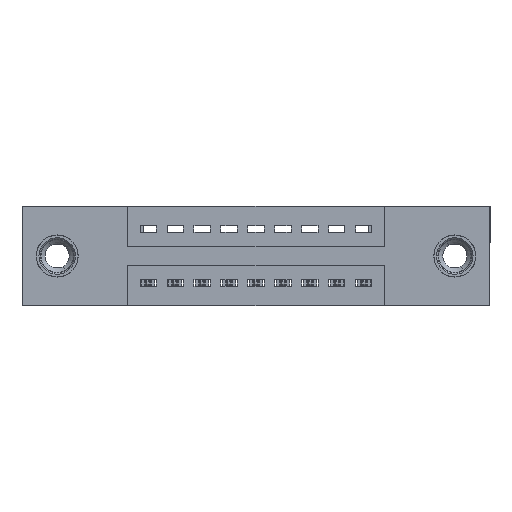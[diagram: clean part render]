
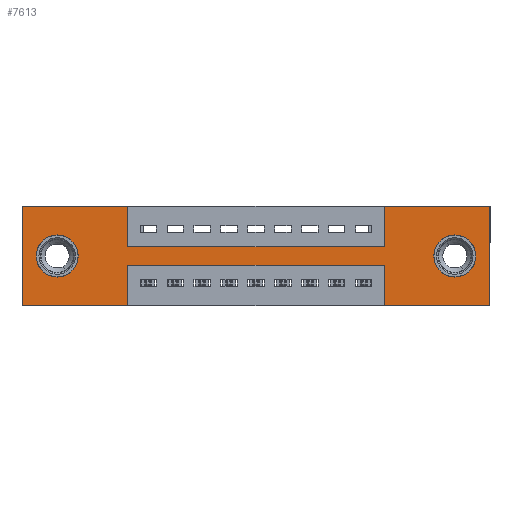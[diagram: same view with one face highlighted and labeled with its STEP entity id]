
A CAD part, front view. The second image highlights one B-rep face of the part: STEP entity #7613.
In plain terms, the highlighted planar face has unit normal (0, -1, 0).
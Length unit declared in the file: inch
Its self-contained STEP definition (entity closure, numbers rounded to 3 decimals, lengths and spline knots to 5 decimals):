
#15 = CARTESIAN_POINT ( 'NONE',  ( 1.735, 0., 0. ) ) ;
#44 = CARTESIAN_POINT ( 'NONE',  ( 1.3425, 0., 0. ) ) ;
#222 = VERTEX_POINT ( 'NONE', #3016 ) ;
#335 = CIRCLE ( 'NONE', #14240, 0.078 ) ;
#431 = ORIENTED_EDGE ( 'NONE', *, *, #9362, .F. ) ;
#639 = CARTESIAN_POINT ( 'NONE',  ( 0., 0., -0.37 ) ) ;
#922 = CARTESIAN_POINT ( 'NONE',  ( 0.3925, 0., -0.22 ) ) ;
#1216 = DIRECTION ( 'NONE',  ( 1., 0., 0. ) ) ;
#1269 = VECTOR ( 'NONE', #6002, 39.37008 ) ;
#1308 = CARTESIAN_POINT ( 'NONE',  ( 0.3925, 0., -0.15 ) ) ;
#1336 = VERTEX_POINT ( 'NONE', #7496 ) ;
#1458 = VECTOR ( 'NONE', #15232, 39.37008 ) ;
#1482 = DIRECTION ( 'NONE',  ( 1., 0., 0. ) ) ;
#1584 = CARTESIAN_POINT ( 'NONE',  ( 1.3425, 0., -0.22 ) ) ;
#1608 = DIRECTION ( 'NONE',  ( 0., 0., -1. ) ) ;
#1689 = VECTOR ( 'NONE', #1216, 39.37008 ) ;
#1743 = EDGE_LOOP ( 'NONE', ( #9976, #431, #6029, #9812, #10681, #13553, #12964, #8786, #4353, #11119, #15261, #13139 ) ) ;
#1906 = DIRECTION ( 'NONE',  ( 0., 0., -1. ) ) ;
#2074 = EDGE_CURVE ( 'NONE', #222, #5820, #11441, .T. ) ;
#2154 = VERTEX_POINT ( 'NONE', #2662 ) ;
#2436 = LINE ( 'NONE', #4130, #11143 ) ;
#2511 = AXIS2_PLACEMENT_3D ( 'NONE', #11464, #7751, #1608 ) ;
#2662 = CARTESIAN_POINT ( 'NONE',  ( 0.3925, 0., -0.37 ) ) ;
#2693 = VERTEX_POINT ( 'NONE', #15 ) ;
#2773 = CARTESIAN_POINT ( 'NONE',  ( 1.605, 0., -0.107 ) ) ;
#2829 = DIRECTION ( 'NONE',  ( 0., 1., 0. ) ) ;
#2889 = CARTESIAN_POINT ( 'NONE',  ( 0., 0., -0.37 ) ) ;
#2910 = VECTOR ( 'NONE', #9819, 39.37008 ) ;
#3016 = CARTESIAN_POINT ( 'NONE',  ( 0., 0., -0.37 ) ) ;
#3171 = DIRECTION ( 'NONE',  ( 0., 1., 0. ) ) ;
#3197 = EDGE_CURVE ( 'NONE', #4443, #6578, #4858, .T. ) ;
#3359 = CARTESIAN_POINT ( 'NONE',  ( 0., 0., 0. ) ) ;
#3431 = EDGE_CURVE ( 'NONE', #7733, #14999, #6390, .T. ) ;
#3702 = CARTESIAN_POINT ( 'NONE',  ( 0., 0., -0.37 ) ) ;
#3777 = EDGE_LOOP ( 'NONE', ( #7436, #11347 ) ) ;
#4051 = CARTESIAN_POINT ( 'NONE',  ( 1.735, 0., -0.37 ) ) ;
#4130 = CARTESIAN_POINT ( 'NONE',  ( 0.3925, 0., -0.22 ) ) ;
#4353 = ORIENTED_EDGE ( 'NONE', *, *, #8789, .F. ) ;
#4442 = VERTEX_POINT ( 'NONE', #4051 ) ;
#4443 = VERTEX_POINT ( 'NONE', #12386 ) ;
#4540 = CARTESIAN_POINT ( 'NONE',  ( 0.13, 0., -0.185 ) ) ;
#4858 = LINE ( 'NONE', #15889, #11058 ) ;
#5031 = EDGE_CURVE ( 'NONE', #14999, #7733, #13100, .T. ) ;
#5149 = VECTOR ( 'NONE', #10310, 39.37008 ) ;
#5389 = AXIS2_PLACEMENT_3D ( 'NONE', #10359, #2829, #9086 ) ;
#5820 = VERTEX_POINT ( 'NONE', #6894 ) ;
#5849 = VECTOR ( 'NONE', #8696, 39.37008 ) ;
#5965 = EDGE_CURVE ( 'NONE', #2693, #4442, #10970, .T. ) ;
#6002 = DIRECTION ( 'NONE',  ( 1., 0., 0. ) ) ;
#6029 = ORIENTED_EDGE ( 'NONE', *, *, #3197, .F. ) ;
#6390 = CIRCLE ( 'NONE', #10800, 0.078 ) ;
#6408 = CARTESIAN_POINT ( 'NONE',  ( 1.735, 0., 0. ) ) ;
#6427 = VECTOR ( 'NONE', #1482, 39.37008 ) ;
#6474 = VERTEX_POINT ( 'NONE', #7418 ) ;
#6578 = VERTEX_POINT ( 'NONE', #1584 ) ;
#6814 = DIRECTION ( 'NONE',  ( 0., 1., 0. ) ) ;
#6894 = CARTESIAN_POINT ( 'NONE',  ( 0., 0., 0. ) ) ;
#7035 = EDGE_CURVE ( 'NONE', #1336, #14138, #335, .T. ) ;
#7060 = EDGE_CURVE ( 'NONE', #2154, #222, #15079, .T. ) ;
#7265 = CARTESIAN_POINT ( 'NONE',  ( 0.3925, 0., -0.15 ) ) ;
#7308 = CARTESIAN_POINT ( 'NONE',  ( 0., 0., 0. ) ) ;
#7373 = EDGE_CURVE ( 'NONE', #13122, #2154, #9649, .T. ) ;
#7418 = CARTESIAN_POINT ( 'NONE',  ( 1.3425, 0., -0.15 ) ) ;
#7436 = ORIENTED_EDGE ( 'NONE', *, *, #5031, .T. ) ;
#7496 = CARTESIAN_POINT ( 'NONE',  ( 0.13, 0., -0.107 ) ) ;
#7502 = VECTOR ( 'NONE', #15582, 39.37008 ) ;
#7613 = ADVANCED_FACE ( 'NONE', ( #9237, #12530, #15632 ), #13455, .T. ) ;
#7733 = VERTEX_POINT ( 'NONE', #9724 ) ;
#7751 = DIRECTION ( 'NONE',  ( 0., 1., 0. ) ) ;
#7794 = EDGE_CURVE ( 'NONE', #9930, #2693, #14861, .T. ) ;
#7814 = DIRECTION ( 'NONE',  ( -1., 0., 0. ) ) ;
#7892 = ORIENTED_EDGE ( 'NONE', *, *, #7035, .T. ) ;
#8064 = DIRECTION ( 'NONE',  ( 0., 0., -1. ) ) ;
#8379 = CARTESIAN_POINT ( 'NONE',  ( 0.3925, 0., 0. ) ) ;
#8553 = CARTESIAN_POINT ( 'NONE',  ( 0., 0., 0. ) ) ;
#8696 = DIRECTION ( 'NONE',  ( 0., 0., 1. ) ) ;
#8786 = ORIENTED_EDGE ( 'NONE', *, *, #11155, .F. ) ;
#8789 = EDGE_CURVE ( 'NONE', #11816, #14502, #13473, .T. ) ;
#8803 = EDGE_CURVE ( 'NONE', #4442, #4443, #12499, .T. ) ;
#9086 = DIRECTION ( 'NONE',  ( 0., 0., 1. ) ) ;
#9162 = EDGE_CURVE ( 'NONE', #5820, #11816, #9972, .T. ) ;
#9237 = FACE_BOUND ( 'NONE', #3777, .T. ) ;
#9283 = CARTESIAN_POINT ( 'NONE',  ( 1.605, 0., -0.185 ) ) ;
#9362 = EDGE_CURVE ( 'NONE', #6578, #13122, #2436, .T. ) ;
#9373 = CARTESIAN_POINT ( 'NONE',  ( 0.3925, 0., -0.37 ) ) ;
#9649 = LINE ( 'NONE', #9373, #12363 ) ;
#9724 = CARTESIAN_POINT ( 'NONE',  ( 1.605, 0., -0.263 ) ) ;
#9812 = ORIENTED_EDGE ( 'NONE', *, *, #8803, .F. ) ;
#9819 = DIRECTION ( 'NONE',  ( 0., 0., 1. ) ) ;
#9930 = VERTEX_POINT ( 'NONE', #15405 ) ;
#9972 = LINE ( 'NONE', #3359, #1269 ) ;
#9976 = ORIENTED_EDGE ( 'NONE', *, *, #7373, .F. ) ;
#10310 = DIRECTION ( 'NONE',  ( 0., 0., -1. ) ) ;
#10359 = CARTESIAN_POINT ( 'NONE',  ( 0.13, 0., -0.185 ) ) ;
#10569 = VECTOR ( 'NONE', #15053, 39.37008 ) ;
#10663 = LINE ( 'NONE', #44, #5849 ) ;
#10681 = ORIENTED_EDGE ( 'NONE', *, *, #5965, .F. ) ;
#10800 = AXIS2_PLACEMENT_3D ( 'NONE', #9283, #3171, #8064 ) ;
#10970 = LINE ( 'NONE', #6408, #10569 ) ;
#11058 = VECTOR ( 'NONE', #12574, 39.37008 ) ;
#11119 = ORIENTED_EDGE ( 'NONE', *, *, #9162, .F. ) ;
#11143 = VECTOR ( 'NONE', #7814, 39.37008 ) ;
#11155 = EDGE_CURVE ( 'NONE', #14502, #6474, #13767, .T. ) ;
#11347 = ORIENTED_EDGE ( 'NONE', *, *, #3431, .T. ) ;
#11441 = LINE ( 'NONE', #8553, #2910 ) ;
#11464 = CARTESIAN_POINT ( 'NONE',  ( 1.605, 0., -0.185 ) ) ;
#11651 = CARTESIAN_POINT ( 'NONE',  ( 0.13, 0., -0.263 ) ) ;
#11816 = VERTEX_POINT ( 'NONE', #8379 ) ;
#11953 = CIRCLE ( 'NONE', #5389, 0.078 ) ;
#12142 = EDGE_CURVE ( 'NONE', #6474, #9930, #10663, .T. ) ;
#12359 = DIRECTION ( 'NONE',  ( 0., -1., 0. ) ) ;
#12363 = VECTOR ( 'NONE', #1906, 39.37008 ) ;
#12386 = CARTESIAN_POINT ( 'NONE',  ( 1.3425, 0., -0.37 ) ) ;
#12499 = LINE ( 'NONE', #2889, #1458 ) ;
#12516 = ORIENTED_EDGE ( 'NONE', *, *, #14030, .T. ) ;
#12530 = FACE_BOUND ( 'NONE', #12541, .T. ) ;
#12541 = EDGE_LOOP ( 'NONE', ( #7892, #12516 ) ) ;
#12574 = DIRECTION ( 'NONE',  ( 0., 0., 1. ) ) ;
#12964 = ORIENTED_EDGE ( 'NONE', *, *, #12142, .F. ) ;
#13083 = DIRECTION ( 'NONE',  ( 0., 0., 1. ) ) ;
#13100 = CIRCLE ( 'NONE', #2511, 0.078 ) ;
#13122 = VERTEX_POINT ( 'NONE', #922 ) ;
#13139 = ORIENTED_EDGE ( 'NONE', *, *, #7060, .F. ) ;
#13397 = DIRECTION ( 'NONE',  ( 0., 0., -1. ) ) ;
#13455 = PLANE ( 'NONE',  #13471 ) ;
#13471 = AXIS2_PLACEMENT_3D ( 'NONE', #3702, #12359, #13397 ) ;
#13473 = LINE ( 'NONE', #15126, #5149 ) ;
#13553 = ORIENTED_EDGE ( 'NONE', *, *, #7794, .F. ) ;
#13767 = LINE ( 'NONE', #7265, #6427 ) ;
#14030 = EDGE_CURVE ( 'NONE', #14138, #1336, #11953, .T. ) ;
#14138 = VERTEX_POINT ( 'NONE', #11651 ) ;
#14240 = AXIS2_PLACEMENT_3D ( 'NONE', #4540, #6814, #13083 ) ;
#14502 = VERTEX_POINT ( 'NONE', #1308 ) ;
#14861 = LINE ( 'NONE', #7308, #1689 ) ;
#14999 = VERTEX_POINT ( 'NONE', #2773 ) ;
#15053 = DIRECTION ( 'NONE',  ( 0., 0., -1. ) ) ;
#15079 = LINE ( 'NONE', #639, #7502 ) ;
#15126 = CARTESIAN_POINT ( 'NONE',  ( 0.3925, 0., 0. ) ) ;
#15232 = DIRECTION ( 'NONE',  ( -1., 0., 0. ) ) ;
#15261 = ORIENTED_EDGE ( 'NONE', *, *, #2074, .F. ) ;
#15405 = CARTESIAN_POINT ( 'NONE',  ( 1.3425, 0., 0. ) ) ;
#15582 = DIRECTION ( 'NONE',  ( -1., 0., 0. ) ) ;
#15632 = FACE_OUTER_BOUND ( 'NONE', #1743, .T. ) ;
#15889 = CARTESIAN_POINT ( 'NONE',  ( 1.3425, 0., -0.37 ) ) ;
